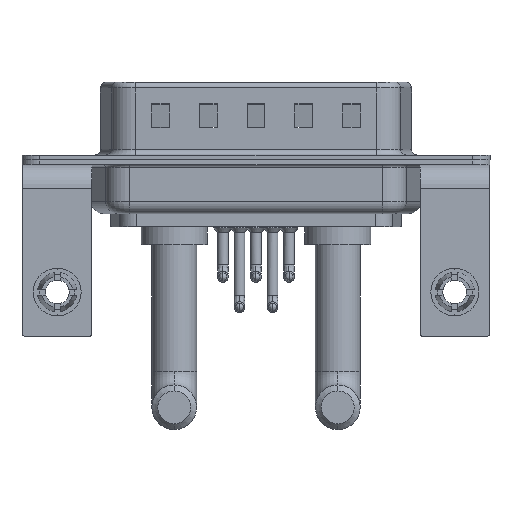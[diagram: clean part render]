
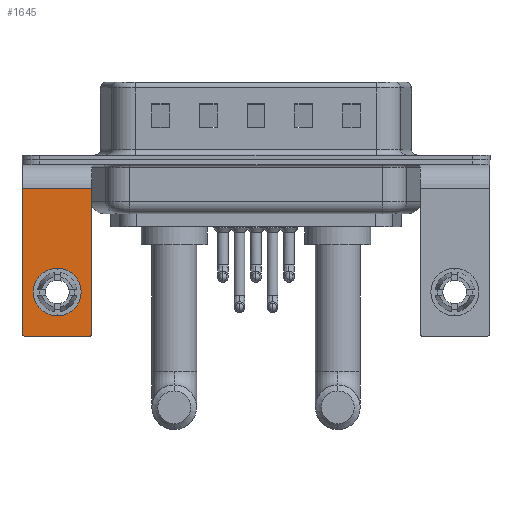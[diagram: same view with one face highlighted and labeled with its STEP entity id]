
A CAD part, front view. The second image highlights one B-rep face of the part: STEP entity #1645.
In plain terms, the highlighted planar face has unit normal (0, -1, 0).
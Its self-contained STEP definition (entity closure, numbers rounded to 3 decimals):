
#513 = LINE ( 'NONE', #16819, #7508 ) ;
#763 = ORIENTED_EDGE ( 'NONE', *, *, #6546, .F. ) ;
#924 = CARTESIAN_POINT ( 'NONE',  ( 2.9, -6.25, -2.4 ) ) ;
#1582 = VERTEX_POINT ( 'NONE', #21395 ) ;
#1645 = ADVANCED_FACE ( 'NONE', ( #6364, #19343 ), #21002, .F. ) ;
#1987 = CARTESIAN_POINT ( 'NONE',  ( -2.9, -6.25, -2.4 ) ) ;
#2137 = DIRECTION ( 'NONE',  ( 0., 0., -1. ) ) ;
#2711 = ORIENTED_EDGE ( 'NONE', *, *, #22632, .T. ) ;
#2850 = DIRECTION ( 'NONE',  ( -1., 0., 0. ) ) ;
#3219 = VERTEX_POINT ( 'NONE', #6739 ) ;
#3633 = CARTESIAN_POINT ( 'NONE',  ( 0., -6.25, -9.07 ) ) ;
#4121 = EDGE_CURVE ( 'NONE', #17317, #12386, #18630, .T. ) ;
#4598 = EDGE_CURVE ( 'NONE', #15459, #14571, #15622, .T. ) ;
#4849 = CARTESIAN_POINT ( 'NONE',  ( 0., -6.25, -11.07 ) ) ;
#4911 = CARTESIAN_POINT ( 'NONE',  ( 2.9, -6.25, -2.4 ) ) ;
#5735 = CARTESIAN_POINT ( 'NONE',  ( 2.65, -6.25, -14.8 ) ) ;
#5986 = EDGE_LOOP ( 'NONE', ( #21213, #10084, #763, #7344, #13287, #18441 ) ) ;
#6247 = DIRECTION ( 'NONE',  ( 0., 1., 0. ) ) ;
#6364 = FACE_BOUND ( 'NONE', #13098, .T. ) ;
#6429 = LINE ( 'NONE', #10226, #10602 ) ;
#6458 = DIRECTION ( 'NONE',  ( -1., 0., 0. ) ) ;
#6546 = EDGE_CURVE ( 'NONE', #15459, #1582, #6429, .T. ) ;
#6692 = LINE ( 'NONE', #4911, #11215 ) ;
#6739 = CARTESIAN_POINT ( 'NONE',  ( -2.9, -6.25, -14.55 ) ) ;
#7344 = ORIENTED_EDGE ( 'NONE', *, *, #4598, .T. ) ;
#7508 = VECTOR ( 'NONE', #18825, 1000. ) ;
#7979 = AXIS2_PLACEMENT_3D ( 'NONE', #4849, #22678, #8543 ) ;
#8177 = CARTESIAN_POINT ( 'NONE',  ( 2.65, -6.25, -14.55 ) ) ;
#8543 = DIRECTION ( 'NONE',  ( 0., 0., 1. ) ) ;
#8679 = DIRECTION ( 'NONE',  ( 0., 0., 1. ) ) ;
#8807 = AXIS2_PLACEMENT_3D ( 'NONE', #22532, #18846, #9339 ) ;
#9339 = DIRECTION ( 'NONE',  ( 0., 0., 1. ) ) ;
#9936 = DIRECTION ( 'NONE',  ( 0., 0., 1. ) ) ;
#10084 = ORIENTED_EDGE ( 'NONE', *, *, #16779, .T. ) ;
#10226 = CARTESIAN_POINT ( 'NONE',  ( 2.9, -6.25, -14.8 ) ) ;
#10602 = VECTOR ( 'NONE', #2850, 1000. ) ;
#11215 = VECTOR ( 'NONE', #6458, 1000. ) ;
#11460 = CARTESIAN_POINT ( 'NONE',  ( 0., -6.25, -13.07 ) ) ;
#12102 = DIRECTION ( 'NONE',  ( 0., 0., 1. ) ) ;
#12386 = VERTEX_POINT ( 'NONE', #3633 ) ;
#12513 = EDGE_CURVE ( 'NONE', #21260, #14914, #6692, .T. ) ;
#12754 = CARTESIAN_POINT ( 'NONE',  ( -2.9, -6.25, -2.4 ) ) ;
#13073 = AXIS2_PLACEMENT_3D ( 'NONE', #17311, #6247, #9936 ) ;
#13098 = EDGE_LOOP ( 'NONE', ( #19859, #2711 ) ) ;
#13287 = ORIENTED_EDGE ( 'NONE', *, *, #18684, .F. ) ;
#14571 = VERTEX_POINT ( 'NONE', #18440 ) ;
#14660 = LINE ( 'NONE', #12754, #18156 ) ;
#14914 = VERTEX_POINT ( 'NONE', #1987 ) ;
#15459 = VERTEX_POINT ( 'NONE', #5735 ) ;
#15588 = DIRECTION ( 'NONE',  ( 0., 1., 0. ) ) ;
#15622 = CIRCLE ( 'NONE', #18652, 0.25 ) ;
#16779 = EDGE_CURVE ( 'NONE', #3219, #1582, #22858, .T. ) ;
#16819 = CARTESIAN_POINT ( 'NONE',  ( 2.9, -6.25, -2.4 ) ) ;
#17311 = CARTESIAN_POINT ( 'NONE',  ( 2.9, -6.25, -2.4 ) ) ;
#17317 = VERTEX_POINT ( 'NONE', #11460 ) ;
#18156 = VECTOR ( 'NONE', #2137, 1000. ) ;
#18249 = CIRCLE ( 'NONE', #7979, 2. ) ;
#18440 = CARTESIAN_POINT ( 'NONE',  ( 2.9, -6.25, -14.55 ) ) ;
#18441 = ORIENTED_EDGE ( 'NONE', *, *, #12513, .T. ) ;
#18630 = CIRCLE ( 'NONE', #21665, 2. ) ;
#18652 = AXIS2_PLACEMENT_3D ( 'NONE', #8177, #22802, #12102 ) ;
#18684 = EDGE_CURVE ( 'NONE', #21260, #14571, #513, .T. ) ;
#18825 = DIRECTION ( 'NONE',  ( 0., 0., -1. ) ) ;
#18846 = DIRECTION ( 'NONE',  ( 0., -1., 0. ) ) ;
#19343 = FACE_OUTER_BOUND ( 'NONE', #5986, .T. ) ;
#19859 = ORIENTED_EDGE ( 'NONE', *, *, #4121, .T. ) ;
#20432 = EDGE_CURVE ( 'NONE', #14914, #3219, #14660, .T. ) ;
#21002 = PLANE ( 'NONE',  #13073 ) ;
#21213 = ORIENTED_EDGE ( 'NONE', *, *, #20432, .T. ) ;
#21260 = VERTEX_POINT ( 'NONE', #924 ) ;
#21395 = CARTESIAN_POINT ( 'NONE',  ( -2.65, -6.25, -14.8 ) ) ;
#21665 = AXIS2_PLACEMENT_3D ( 'NONE', #23169, #15588, #8679 ) ;
#22532 = CARTESIAN_POINT ( 'NONE',  ( -2.65, -6.25, -14.55 ) ) ;
#22632 = EDGE_CURVE ( 'NONE', #12386, #17317, #18249, .T. ) ;
#22678 = DIRECTION ( 'NONE',  ( 0., 1., 0. ) ) ;
#22802 = DIRECTION ( 'NONE',  ( 0., -1., 0. ) ) ;
#22858 = CIRCLE ( 'NONE', #8807, 0.25 ) ;
#23169 = CARTESIAN_POINT ( 'NONE',  ( 0., -6.25, -11.07 ) ) ;
